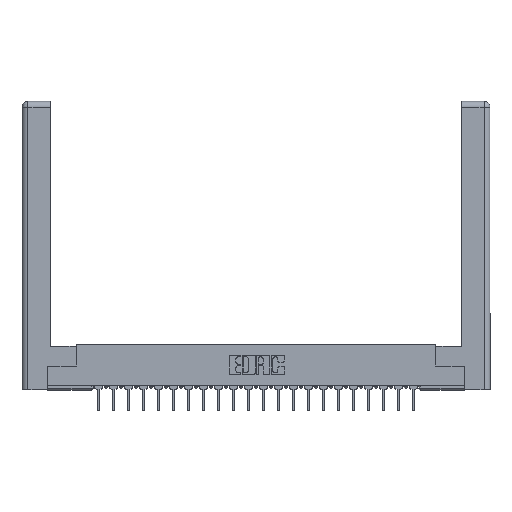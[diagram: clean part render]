
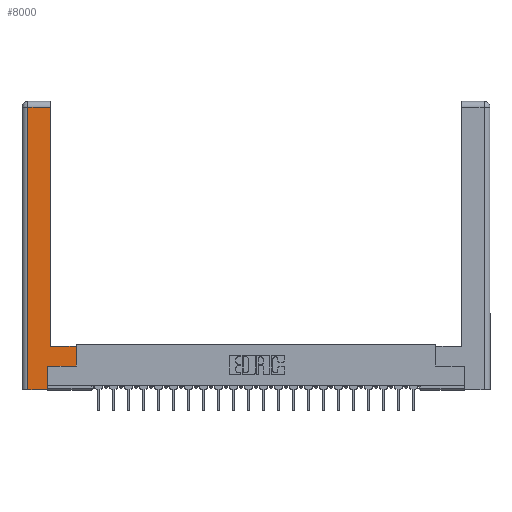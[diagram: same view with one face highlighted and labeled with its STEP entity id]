
A CAD part, top view. The second image highlights one B-rep face of the part: STEP entity #8000.
In plain terms, the highlighted planar face has unit normal (0, 0, 1).
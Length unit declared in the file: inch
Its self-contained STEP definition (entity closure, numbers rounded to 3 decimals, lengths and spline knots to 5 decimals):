
#74 = EDGE_CURVE ( 'NONE', #4960, #5555, #22121, .T. ) ;
#1224 = EDGE_CURVE ( 'NONE', #5555, #19450, #20726, .T. ) ;
#1526 = CARTESIAN_POINT ( 'NONE',  ( 0.265, 0.245, 0. ) ) ;
#2272 = ORIENTED_EDGE ( 'NONE', *, *, #20060, .T. ) ;
#2587 = DIRECTION ( 'NONE',  ( 1., 0., 0. ) ) ;
#3658 = VECTOR ( 'NONE', #2587, 39.37008 ) ;
#3692 = AXIS2_PLACEMENT_3D ( 'NONE', #20760, #4166, #10311 ) ;
#3952 = CARTESIAN_POINT ( 'NONE',  ( 0.295, 3., 0. ) ) ;
#4132 = DIRECTION ( 'NONE',  ( -1., 0., 0. ) ) ;
#4166 = DIRECTION ( 'NONE',  ( 0., 0., -1. ) ) ;
#4350 = EDGE_CURVE ( 'NONE', #21632, #8430, #20440, .T. ) ;
#4725 = DIRECTION ( 'NONE',  ( 0., 1., 0. ) ) ;
#4832 = CARTESIAN_POINT ( 'NONE',  ( 0.265, 0.245, 0. ) ) ;
#4875 = ORIENTED_EDGE ( 'NONE', *, *, #74, .T. ) ;
#4960 = VERTEX_POINT ( 'NONE', #6135 ) ;
#5069 = CARTESIAN_POINT ( 'NONE',  ( 0.0615, 2.94, 0. ) ) ;
#5100 = CARTESIAN_POINT ( 'NONE',  ( 0.565, 0.45, 0. ) ) ;
#5461 = ORIENTED_EDGE ( 'NONE', *, *, #4350, .T. ) ;
#5555 = VERTEX_POINT ( 'NONE', #23476 ) ;
#5568 = DIRECTION ( 'NONE',  ( 0., 1., 0. ) ) ;
#6003 = FACE_OUTER_BOUND ( 'NONE', #17534, .T. ) ;
#6135 = CARTESIAN_POINT ( 'NONE',  ( 0.295, 0.45, 0. ) ) ;
#6171 = EDGE_CURVE ( 'NONE', #19450, #15867, #16782, .T. ) ;
#6350 = VECTOR ( 'NONE', #7243, 39.37008 ) ;
#7046 = DIRECTION ( 'NONE',  ( 1., 0., 0. ) ) ;
#7114 = ORIENTED_EDGE ( 'NONE', *, *, #17726, .T. ) ;
#7243 = DIRECTION ( 'NONE',  ( 0., -1., 0. ) ) ;
#7457 = DIRECTION ( 'NONE',  ( -1., 0., 0. ) ) ;
#7705 = VECTOR ( 'NONE', #5568, 39.37008 ) ;
#7974 = LINE ( 'NONE', #20895, #3658 ) ;
#8000 = ADVANCED_FACE ( 'NONE', ( #6003 ), #13369, .F. ) ;
#8091 = CARTESIAN_POINT ( 'NONE',  ( 0.565, 0.45, 0. ) ) ;
#8430 = VERTEX_POINT ( 'NONE', #4832 ) ;
#8441 = CARTESIAN_POINT ( 'NONE',  ( 0.265, 0., 0. ) ) ;
#8620 = VECTOR ( 'NONE', #7046, 39.37008 ) ;
#9152 = CARTESIAN_POINT ( 'NONE',  ( 0.295, 0.45, 0. ) ) ;
#10311 = DIRECTION ( 'NONE',  ( -1., 0., 0. ) ) ;
#10514 = ORIENTED_EDGE ( 'NONE', *, *, #22513, .T. ) ;
#10812 = LINE ( 'NONE', #9152, #13000 ) ;
#11030 = CARTESIAN_POINT ( 'NONE',  ( 0.0615, 2.94, 0. ) ) ;
#12145 = VECTOR ( 'NONE', #4725, 39.37008 ) ;
#13000 = VECTOR ( 'NONE', #7457, 39.37008 ) ;
#13369 = PLANE ( 'NONE',  #3692 ) ;
#14057 = CARTESIAN_POINT ( 'NONE',  ( 0.565, 0.245, 0. ) ) ;
#15754 = ORIENTED_EDGE ( 'NONE', *, *, #1224, .T. ) ;
#15867 = VERTEX_POINT ( 'NONE', #20333 ) ;
#16200 = LINE ( 'NONE', #5100, #12145 ) ;
#16439 = ORIENTED_EDGE ( 'NONE', *, *, #18449, .T. ) ;
#16782 = LINE ( 'NONE', #21887, #6350 ) ;
#17534 = EDGE_LOOP ( 'NONE', ( #4875, #15754, #22350, #16439, #5461, #10514, #7114, #2272 ) ) ;
#17726 = EDGE_CURVE ( 'NONE', #19906, #19753, #16200, .T. ) ;
#18449 = EDGE_CURVE ( 'NONE', #15867, #21632, #7974, .T. ) ;
#19450 = VERTEX_POINT ( 'NONE', #5069 ) ;
#19753 = VERTEX_POINT ( 'NONE', #8091 ) ;
#19859 = LINE ( 'NONE', #14057, #8620 ) ;
#19906 = VERTEX_POINT ( 'NONE', #21500 ) ;
#20060 = EDGE_CURVE ( 'NONE', #19753, #4960, #10812, .T. ) ;
#20333 = CARTESIAN_POINT ( 'NONE',  ( 0.0615, 0., 0. ) ) ;
#20440 = LINE ( 'NONE', #1526, #7705 ) ;
#20530 = DIRECTION ( 'NONE',  ( 0., 1., 0. ) ) ;
#20726 = LINE ( 'NONE', #11030, #22496 ) ;
#20760 = CARTESIAN_POINT ( 'NONE',  ( 0., 0., 0. ) ) ;
#20895 = CARTESIAN_POINT ( 'NONE',  ( 0.265, 0., 0. ) ) ;
#21500 = CARTESIAN_POINT ( 'NONE',  ( 0.565, 0.245, 0. ) ) ;
#21632 = VERTEX_POINT ( 'NONE', #8441 ) ;
#21887 = CARTESIAN_POINT ( 'NONE',  ( 0.0615, 0., 0. ) ) ;
#22084 = VECTOR ( 'NONE', #20530, 39.37008 ) ;
#22121 = LINE ( 'NONE', #3952, #22084 ) ;
#22350 = ORIENTED_EDGE ( 'NONE', *, *, #6171, .T. ) ;
#22496 = VECTOR ( 'NONE', #4132, 39.37008 ) ;
#22513 = EDGE_CURVE ( 'NONE', #8430, #19906, #19859, .T. ) ;
#23476 = CARTESIAN_POINT ( 'NONE',  ( 0.295, 2.94, 0. ) ) ;
